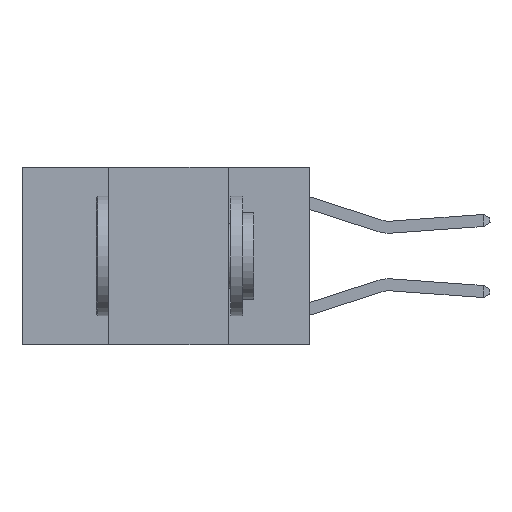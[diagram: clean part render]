
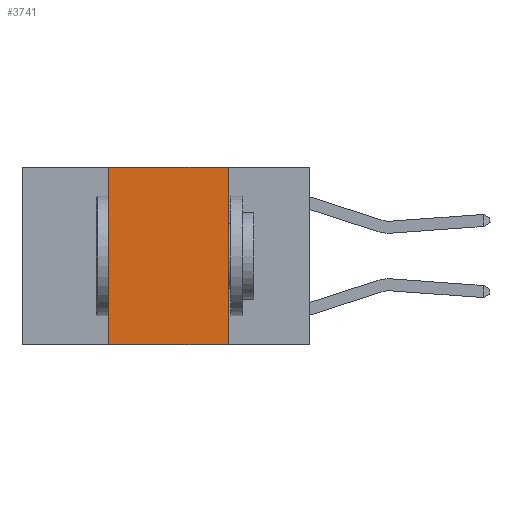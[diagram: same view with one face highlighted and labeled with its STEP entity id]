
A CAD part, left-side view. The second image highlights one B-rep face of the part: STEP entity #3741.
In plain terms, the highlighted planar face has unit normal (-1, 0, 0).
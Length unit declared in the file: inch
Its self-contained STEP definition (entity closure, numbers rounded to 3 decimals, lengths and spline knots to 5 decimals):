
#62 = EDGE_CURVE ( 'NONE', #3595, #8026, #3818, .T. ) ;
#550 = VECTOR ( 'NONE', #6363, 39.37008 ) ;
#820 = DIRECTION ( 'NONE',  ( 1., 0., 0. ) ) ;
#2057 = ORIENTED_EDGE ( 'NONE', *, *, #8171, .F. ) ;
#2381 = EDGE_CURVE ( 'NONE', #7868, #8026, #3073, .T. ) ;
#2782 = VECTOR ( 'NONE', #10695, 39.37008 ) ;
#3073 = LINE ( 'NONE', #4631, #550 ) ;
#3595 = VERTEX_POINT ( 'NONE', #7382 ) ;
#3741 = ADVANCED_FACE ( 'NONE', ( #4285 ), #10104, .F. ) ;
#3818 = LINE ( 'NONE', #7244, #2782 ) ;
#3922 = AXIS2_PLACEMENT_3D ( 'NONE', #10318, #820, #6762 ) ;
#4156 = CARTESIAN_POINT ( 'NONE',  ( 0., 0.42, 0. ) ) ;
#4276 = LINE ( 'NONE', #5862, #4986 ) ;
#4285 = FACE_OUTER_BOUND ( 'NONE', #9717, .T. ) ;
#4631 = CARTESIAN_POINT ( 'NONE',  ( 0., 0.6, -0.37 ) ) ;
#4940 = DIRECTION ( 'NONE',  ( 0., -1., 0. ) ) ;
#4986 = VECTOR ( 'NONE', #4940, 39.37008 ) ;
#5292 = CARTESIAN_POINT ( 'NONE',  ( 0., 0.17, -0.37 ) ) ;
#5529 = EDGE_CURVE ( 'NONE', #5749, #3595, #4276, .T. ) ;
#5749 = VERTEX_POINT ( 'NONE', #6177 ) ;
#5862 = CARTESIAN_POINT ( 'NONE',  ( 0., 0.6, 0. ) ) ;
#6177 = CARTESIAN_POINT ( 'NONE',  ( 0., 0.42, 0. ) ) ;
#6363 = DIRECTION ( 'NONE',  ( 0., -1., 0. ) ) ;
#6762 = DIRECTION ( 'NONE',  ( 0., 0., -1. ) ) ;
#7244 = CARTESIAN_POINT ( 'NONE',  ( 0., 0.17, 0. ) ) ;
#7382 = CARTESIAN_POINT ( 'NONE',  ( 0., 0.17, 0. ) ) ;
#7630 = ORIENTED_EDGE ( 'NONE', *, *, #5529, .F. ) ;
#7868 = VERTEX_POINT ( 'NONE', #10273 ) ;
#7985 = ORIENTED_EDGE ( 'NONE', *, *, #62, .F. ) ;
#8026 = VERTEX_POINT ( 'NONE', #5292 ) ;
#8171 = EDGE_CURVE ( 'NONE', #7868, #5749, #10196, .T. ) ;
#8549 = ORIENTED_EDGE ( 'NONE', *, *, #2381, .T. ) ;
#9226 = DIRECTION ( 'NONE',  ( 0., 0., 1. ) ) ;
#9610 = VECTOR ( 'NONE', #9226, 39.37008 ) ;
#9717 = EDGE_LOOP ( 'NONE', ( #7985, #7630, #2057, #8549 ) ) ;
#10104 = PLANE ( 'NONE',  #3922 ) ;
#10196 = LINE ( 'NONE', #4156, #9610 ) ;
#10273 = CARTESIAN_POINT ( 'NONE',  ( 0., 0.42, -0.37 ) ) ;
#10318 = CARTESIAN_POINT ( 'NONE',  ( 0., 0.6, 0. ) ) ;
#10695 = DIRECTION ( 'NONE',  ( 0., 0., -1. ) ) ;
